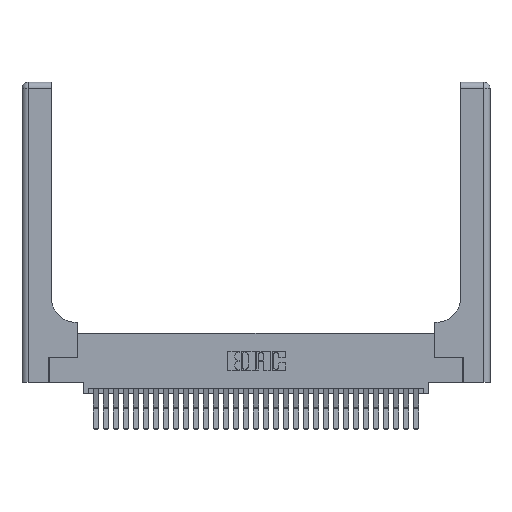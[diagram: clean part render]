
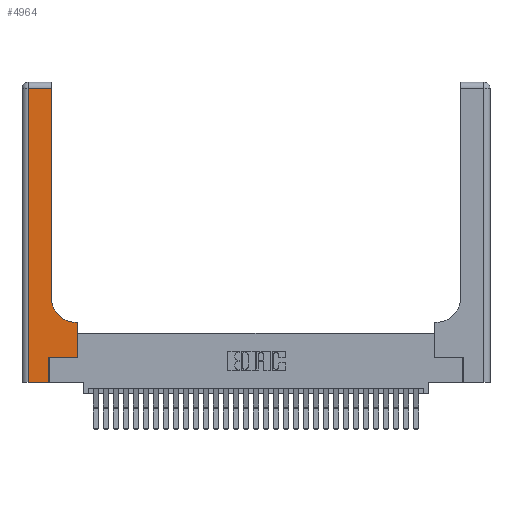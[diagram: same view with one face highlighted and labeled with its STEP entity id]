
A CAD part, top view. The second image highlights one B-rep face of the part: STEP entity #4964.
In plain terms, the highlighted planar face has unit normal (0, 0, 1).
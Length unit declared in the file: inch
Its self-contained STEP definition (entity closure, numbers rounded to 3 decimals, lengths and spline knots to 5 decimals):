
#157 = LINE ( 'NONE', #20492, #6917 ) ;
#411 = VECTOR ( 'NONE', #12985, 39.37008 ) ;
#498 = ORIENTED_EDGE ( 'NONE', *, *, #24752, .T. ) ;
#642 = DIRECTION ( 'NONE',  ( 0., -1., 0. ) ) ;
#877 = ORIENTED_EDGE ( 'NONE', *, *, #14812, .T. ) ;
#976 = CARTESIAN_POINT ( 'NONE',  ( 0.269, 0.25, 0.37 ) ) ;
#1152 = EDGE_CURVE ( 'NONE', #24505, #14828, #24031, .T. ) ;
#2135 = ORIENTED_EDGE ( 'NONE', *, *, #14385, .T. ) ;
#2453 = LINE ( 'NONE', #24556, #15174 ) ;
#2792 = DIRECTION ( 'NONE',  ( 0., 1., 0. ) ) ;
#2812 = CARTESIAN_POINT ( 'NONE',  ( 0.06, 0., 0.37 ) ) ;
#2922 = EDGE_CURVE ( 'NONE', #24531, #12397, #157, .T. ) ;
#2950 = VECTOR ( 'NONE', #642, 39.37008 ) ;
#3600 = FACE_OUTER_BOUND ( 'NONE', #3645, .T. ) ;
#3645 = EDGE_LOOP ( 'NONE', ( #20317, #877, #16018, #18373, #498, #14037, #21508, #2135, #15644 ) ) ;
#4601 = CARTESIAN_POINT ( 'NONE',  ( 0.2915, 2.94, 0.37 ) ) ;
#4964 = ADVANCED_FACE ( 'NONE', ( #3600 ), #23653, .F. ) ;
#5476 = VERTEX_POINT ( 'NONE', #14740 ) ;
#6138 = VERTEX_POINT ( 'NONE', #9762 ) ;
#6341 = LINE ( 'NONE', #25507, #13095 ) ;
#6917 = VECTOR ( 'NONE', #2792, 39.37008 ) ;
#7013 = CARTESIAN_POINT ( 'NONE',  ( 0.5415, 0.6, 0.37 ) ) ;
#7952 = EDGE_CURVE ( 'NONE', #6138, #32362, #22327, .T. ) ;
#8501 = DIRECTION ( 'NONE',  ( 0., 0., -1. ) ) ;
#9218 = VECTOR ( 'NONE', #27199, 39.37008 ) ;
#9575 = CARTESIAN_POINT ( 'NONE',  ( 0.2915, 3., 0.37 ) ) ;
#9762 = CARTESIAN_POINT ( 'NONE',  ( 0.06, 2.94, 0.37 ) ) ;
#10338 = LINE ( 'NONE', #976, #17118 ) ;
#10374 = EDGE_CURVE ( 'NONE', #32362, #30393, #6341, .T. ) ;
#10376 = DIRECTION ( 'NONE',  ( 1., 0., 0. ) ) ;
#10421 = CARTESIAN_POINT ( 'NONE',  ( 0.269, 0., 0.37 ) ) ;
#12218 = CARTESIAN_POINT ( 'NONE',  ( 0.5585, 0.25, 0.37 ) ) ;
#12397 = VERTEX_POINT ( 'NONE', #13441 ) ;
#12985 = DIRECTION ( 'NONE',  ( 0., 1., 0. ) ) ;
#13095 = VECTOR ( 'NONE', #10376, 39.37008 ) ;
#13441 = CARTESIAN_POINT ( 'NONE',  ( 0.5585, 0.6, 0.37 ) ) ;
#14037 = ORIENTED_EDGE ( 'NONE', *, *, #30068, .T. ) ;
#14385 = EDGE_CURVE ( 'NONE', #12397, #24505, #2453, .T. ) ;
#14740 = CARTESIAN_POINT ( 'NONE',  ( 0.269, 0.25, 0.37 ) ) ;
#14812 = EDGE_CURVE ( 'NONE', #20674, #6138, #23377, .T. ) ;
#14828 = VERTEX_POINT ( 'NONE', #23868 ) ;
#15174 = VECTOR ( 'NONE', #27045, 39.37008 ) ;
#15644 = ORIENTED_EDGE ( 'NONE', *, *, #1152, .T. ) ;
#16018 = ORIENTED_EDGE ( 'NONE', *, *, #7952, .T. ) ;
#16104 = CARTESIAN_POINT ( 'NONE',  ( 0., 3., 0.37 ) ) ;
#16220 = DIRECTION ( 'NONE',  ( 1., 0., 0. ) ) ;
#17118 = VECTOR ( 'NONE', #16220, 39.37008 ) ;
#18373 = ORIENTED_EDGE ( 'NONE', *, *, #10374, .T. ) ;
#20317 = ORIENTED_EDGE ( 'NONE', *, *, #29017, .T. ) ;
#20492 = CARTESIAN_POINT ( 'NONE',  ( 0.5585, 0.25, 0.37 ) ) ;
#20674 = VERTEX_POINT ( 'NONE', #4601 ) ;
#20814 = CARTESIAN_POINT ( 'NONE',  ( 0.06, 3., 0.37 ) ) ;
#21508 = ORIENTED_EDGE ( 'NONE', *, *, #2922, .T. ) ;
#21889 = LINE ( 'NONE', #9575, #9218 ) ;
#22327 = LINE ( 'NONE', #20814, #2950 ) ;
#22878 = AXIS2_PLACEMENT_3D ( 'NONE', #16104, #8501, #26172 ) ;
#23377 = LINE ( 'NONE', #31172, #29156 ) ;
#23653 = PLANE ( 'NONE',  #22878 ) ;
#23868 = CARTESIAN_POINT ( 'NONE',  ( 0.2915, 0.85, 0.37 ) ) ;
#24031 = CIRCLE ( 'NONE', #32489, 0.25 ) ;
#24505 = VERTEX_POINT ( 'NONE', #7013 ) ;
#24531 = VERTEX_POINT ( 'NONE', #12218 ) ;
#24556 = CARTESIAN_POINT ( 'NONE',  ( 0.2915, 0.6, 0.37 ) ) ;
#24752 = EDGE_CURVE ( 'NONE', #30393, #5476, #26501, .T. ) ;
#25507 = CARTESIAN_POINT ( 'NONE',  ( 0., 0., 0.37 ) ) ;
#25961 = DIRECTION ( 'NONE',  ( -1., 0., 0. ) ) ;
#26172 = DIRECTION ( 'NONE',  ( -1., 0., 0. ) ) ;
#26501 = LINE ( 'NONE', #10421, #411 ) ;
#27045 = DIRECTION ( 'NONE',  ( -1., 0., 0. ) ) ;
#27199 = DIRECTION ( 'NONE',  ( 0., 1., 0. ) ) ;
#29017 = EDGE_CURVE ( 'NONE', #14828, #20674, #21889, .T. ) ;
#29156 = VECTOR ( 'NONE', #25961, 39.37008 ) ;
#29369 = DIRECTION ( 'NONE',  ( 1., 0., 0. ) ) ;
#29413 = DIRECTION ( 'NONE',  ( 0., 0., -1. ) ) ;
#29479 = CARTESIAN_POINT ( 'NONE',  ( 0.5415, 0.85, 0.37 ) ) ;
#29780 = CARTESIAN_POINT ( 'NONE',  ( 0.269, 0., 0.37 ) ) ;
#30068 = EDGE_CURVE ( 'NONE', #5476, #24531, #10338, .T. ) ;
#30393 = VERTEX_POINT ( 'NONE', #29780 ) ;
#31172 = CARTESIAN_POINT ( 'NONE',  ( 0., 2.94, 0.37 ) ) ;
#32362 = VERTEX_POINT ( 'NONE', #2812 ) ;
#32489 = AXIS2_PLACEMENT_3D ( 'NONE', #29479, #29413, #29369 ) ;
